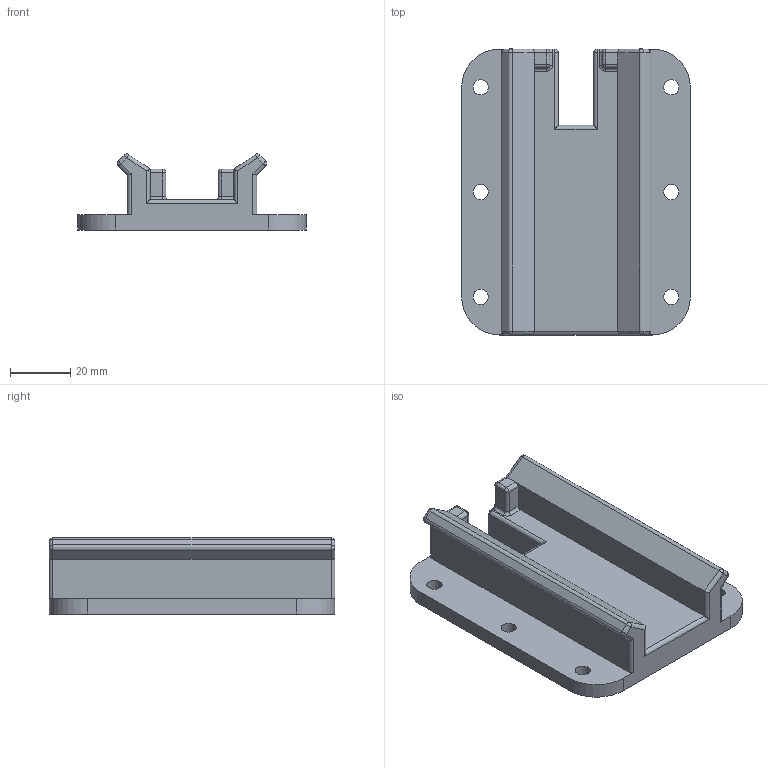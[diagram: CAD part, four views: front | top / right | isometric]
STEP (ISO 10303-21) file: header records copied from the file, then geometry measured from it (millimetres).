
FILE_DESCRIPTION(/* description */ (''),/* implementation_level */ '2;1');
FILE_NAME(/* name */ 'Quickdraw V3 (Enclosed 17 mm barrel Gap).step',/* time_stamp */ '2022-01-04T10:45:27-08:00',/* author */ (''),/* organization */ (''),/* preprocessor_version */ 'ST-DEVELOPER v18.1',/* originating_system */ 'Autodesk Translation Framework v10.10.0.1391',/* authorisation */ '');
FILE_SCHEMA (('AUTOMOTIVE_DESIGN { 1 0 10303 214 3 1 1 }'));
Length unit declared in the file: millimetre
Products named in the file (1): (Unsaved)
Bounding box: 76.2 x 95.25 x 25.33 mm (x, y, z)
Volume: 65540.4 mm3; surface area: 28145.4 mm2
Topology: 1 solids, 3 shells, 106 faces, 249 edges, 142 vertices
Faces by surface type: cylinder 56, plane 32, sphere 8, bspline 6, torus 4
Full cylindrical faces by diameter (mm): 5.08 x6, 32.623 x2
Entity records: 3130 total; most frequent: CARTESIAN_POINT 649, DIRECTION 542, ORIENTED_EDGE 484, EDGE_CURVE 242, AXIS2_PLACEMENT_3D 205, VERTEX_POINT 142, LINE 132, VECTOR 132
